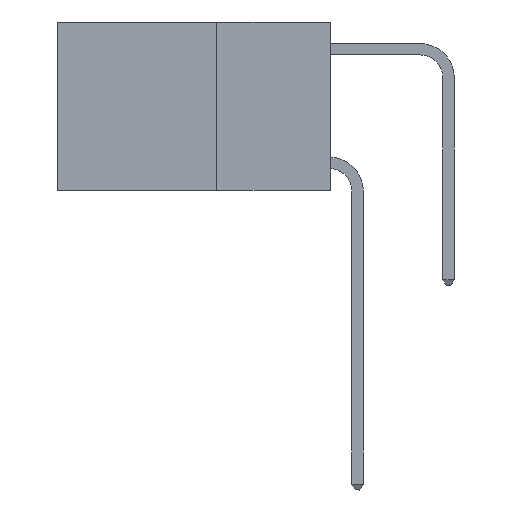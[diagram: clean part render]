
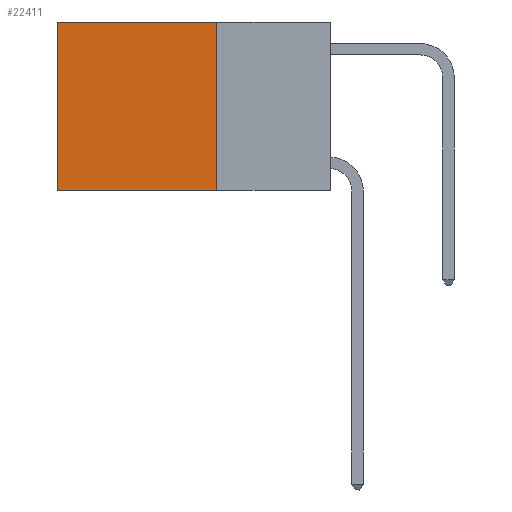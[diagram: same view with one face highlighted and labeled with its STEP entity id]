
A CAD part, left-side view. The second image highlights one B-rep face of the part: STEP entity #22411.
In plain terms, the highlighted planar face has unit normal (-1, 0, 0).
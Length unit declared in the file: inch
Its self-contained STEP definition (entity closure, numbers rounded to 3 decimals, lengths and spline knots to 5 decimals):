
#2427 = VERTEX_POINT ( 'NONE', #13632 ) ;
#3155 = FACE_OUTER_BOUND ( 'NONE', #15002, .T. ) ;
#4202 = LINE ( 'NONE', #4495, #23636 ) ;
#4495 = CARTESIAN_POINT ( 'NONE',  ( 0.2625, 0.25, -0.37 ) ) ;
#4996 = CARTESIAN_POINT ( 'NONE',  ( 0.2625, 0.6, 0. ) ) ;
#5338 = VERTEX_POINT ( 'NONE', #4996 ) ;
#6061 = CARTESIAN_POINT ( 'NONE',  ( 0.2625, 0.25, -0.37 ) ) ;
#6688 = DIRECTION ( 'NONE',  ( 0., 0., -1. ) ) ;
#6954 = EDGE_CURVE ( 'NONE', #19965, #5338, #17425, .T. ) ;
#7794 = DIRECTION ( 'NONE',  ( 1., 0., 0. ) ) ;
#9241 = VECTOR ( 'NONE', #16518, 39.37008 ) ;
#9917 = LINE ( 'NONE', #19073, #9241 ) ;
#10943 = DIRECTION ( 'NONE',  ( 0., 1., 0. ) ) ;
#11389 = EDGE_CURVE ( 'NONE', #19965, #24710, #20920, .T. ) ;
#13632 = CARTESIAN_POINT ( 'NONE',  ( 0.2625, 0.6, -0.37 ) ) ;
#14178 = CARTESIAN_POINT ( 'NONE',  ( 0.2625, 0.25, 0. ) ) ;
#15002 = EDGE_LOOP ( 'NONE', ( #18269, #28757, #18314, #23597 ) ) ;
#16518 = DIRECTION ( 'NONE',  ( 0., 0., -1. ) ) ;
#16934 = DIRECTION ( 'NONE',  ( 0., 0., -1. ) ) ;
#17425 = LINE ( 'NONE', #28844, #28944 ) ;
#18269 = ORIENTED_EDGE ( 'NONE', *, *, #25400, .T. ) ;
#18314 = ORIENTED_EDGE ( 'NONE', *, *, #11389, .F. ) ;
#19073 = CARTESIAN_POINT ( 'NONE',  ( 0.2625, 0.6, 0. ) ) ;
#19193 = CARTESIAN_POINT ( 'NONE',  ( 0.2625, 0.25, 0. ) ) ;
#19475 = VECTOR ( 'NONE', #6688, 39.37008 ) ;
#19965 = VERTEX_POINT ( 'NONE', #20980 ) ;
#20920 = LINE ( 'NONE', #14178, #19475 ) ;
#20980 = CARTESIAN_POINT ( 'NONE',  ( 0.2625, 0.25, 0. ) ) ;
#21454 = PLANE ( 'NONE',  #26843 ) ;
#22411 = ADVANCED_FACE ( 'NONE', ( #3155 ), #21454, .F. ) ;
#23597 = ORIENTED_EDGE ( 'NONE', *, *, #6954, .T. ) ;
#23636 = VECTOR ( 'NONE', #10943, 39.37008 ) ;
#24710 = VERTEX_POINT ( 'NONE', #6061 ) ;
#25400 = EDGE_CURVE ( 'NONE', #5338, #2427, #9917, .T. ) ;
#25724 = EDGE_CURVE ( 'NONE', #24710, #2427, #4202, .T. ) ;
#26605 = DIRECTION ( 'NONE',  ( 0., 1., 0. ) ) ;
#26843 = AXIS2_PLACEMENT_3D ( 'NONE', #19193, #7794, #16934 ) ;
#28757 = ORIENTED_EDGE ( 'NONE', *, *, #25724, .F. ) ;
#28844 = CARTESIAN_POINT ( 'NONE',  ( 0.2625, 0.25, 0. ) ) ;
#28944 = VECTOR ( 'NONE', #26605, 39.37008 ) ;
